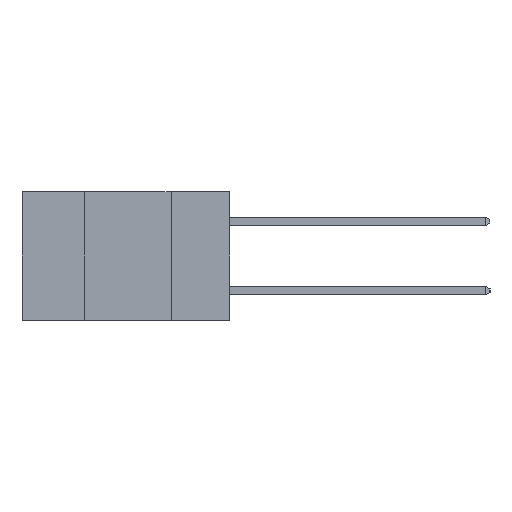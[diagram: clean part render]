
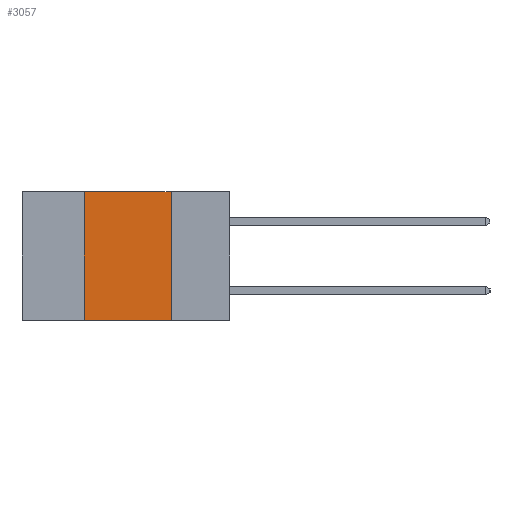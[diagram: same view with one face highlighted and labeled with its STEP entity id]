
A CAD part, left-side view. The second image highlights one B-rep face of the part: STEP entity #3057.
In plain terms, the highlighted planar face has unit normal (-1, 0, 0).
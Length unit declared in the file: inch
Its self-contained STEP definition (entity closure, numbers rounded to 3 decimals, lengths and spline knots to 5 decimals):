
#5 = CARTESIAN_POINT ( 'NONE',  ( 0., 0.42, 0. ) ) ;
#366 = CARTESIAN_POINT ( 'NONE',  ( 0., 0.17, -0.37 ) ) ;
#956 = PLANE ( 'NONE',  #6071 ) ;
#1127 = CARTESIAN_POINT ( 'NONE',  ( 0., 0.6, -0.37 ) ) ;
#1192 = DIRECTION ( 'NONE',  ( 0., 0., -1. ) ) ;
#1648 = DIRECTION ( 'NONE',  ( 1., 0., 0. ) ) ;
#2067 = LINE ( 'NONE', #366, #7387 ) ;
#2118 = EDGE_LOOP ( 'NONE', ( #4561, #7079, #7210, #5428 ) ) ;
#2182 = DIRECTION ( 'NONE',  ( 0., 0., 1. ) ) ;
#3050 = VERTEX_POINT ( 'NONE', #5 ) ;
#3057 = ADVANCED_FACE ( 'NONE', ( #6530 ), #956, .F. ) ;
#3674 = CARTESIAN_POINT ( 'NONE',  ( 0., 0.17, -0.37 ) ) ;
#3709 = CARTESIAN_POINT ( 'NONE',  ( 0., 0.42, -0.37 ) ) ;
#4132 = CARTESIAN_POINT ( 'NONE',  ( 0., 0.42, -0.37 ) ) ;
#4561 = ORIENTED_EDGE ( 'NONE', *, *, #4891, .F. ) ;
#4661 = LINE ( 'NONE', #3709, #6610 ) ;
#4797 = VECTOR ( 'NONE', #8774, 39.37008 ) ;
#4891 = EDGE_CURVE ( 'NONE', #6665, #5450, #2067, .T. ) ;
#5428 = ORIENTED_EDGE ( 'NONE', *, *, #6036, .T. ) ;
#5450 = VERTEX_POINT ( 'NONE', #3674 ) ;
#6036 = EDGE_CURVE ( 'NONE', #6114, #5450, #8378, .T. ) ;
#6071 = AXIS2_PLACEMENT_3D ( 'NONE', #8577, #1648, #6527 ) ;
#6114 = VERTEX_POINT ( 'NONE', #4132 ) ;
#6121 = VECTOR ( 'NONE', #6234, 39.37008 ) ;
#6234 = DIRECTION ( 'NONE',  ( 0., -1., 0. ) ) ;
#6527 = DIRECTION ( 'NONE',  ( 0., 0., -1. ) ) ;
#6530 = FACE_OUTER_BOUND ( 'NONE', #2118, .T. ) ;
#6610 = VECTOR ( 'NONE', #2182, 39.37008 ) ;
#6665 = VERTEX_POINT ( 'NONE', #7183 ) ;
#6849 = CARTESIAN_POINT ( 'NONE',  ( 0., 0.6, 0. ) ) ;
#7079 = ORIENTED_EDGE ( 'NONE', *, *, #7249, .F. ) ;
#7183 = CARTESIAN_POINT ( 'NONE',  ( 0., 0.17, 0. ) ) ;
#7210 = ORIENTED_EDGE ( 'NONE', *, *, #8654, .F. ) ;
#7249 = EDGE_CURVE ( 'NONE', #3050, #6665, #7920, .T. ) ;
#7387 = VECTOR ( 'NONE', #1192, 39.37008 ) ;
#7920 = LINE ( 'NONE', #6849, #6121 ) ;
#8378 = LINE ( 'NONE', #1127, #4797 ) ;
#8577 = CARTESIAN_POINT ( 'NONE',  ( 0., 0.6, 0. ) ) ;
#8654 = EDGE_CURVE ( 'NONE', #6114, #3050, #4661, .T. ) ;
#8774 = DIRECTION ( 'NONE',  ( 0., -1., 0. ) ) ;
